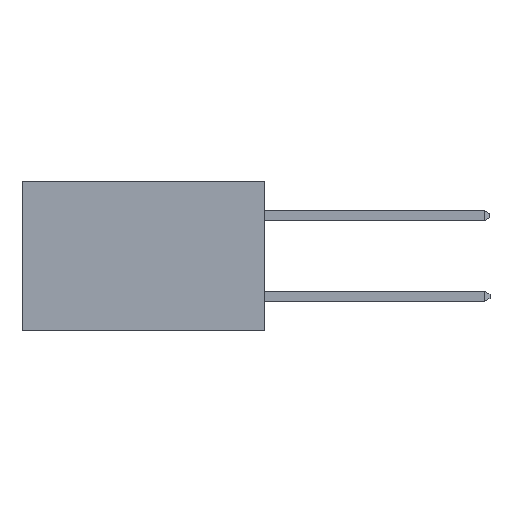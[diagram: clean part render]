
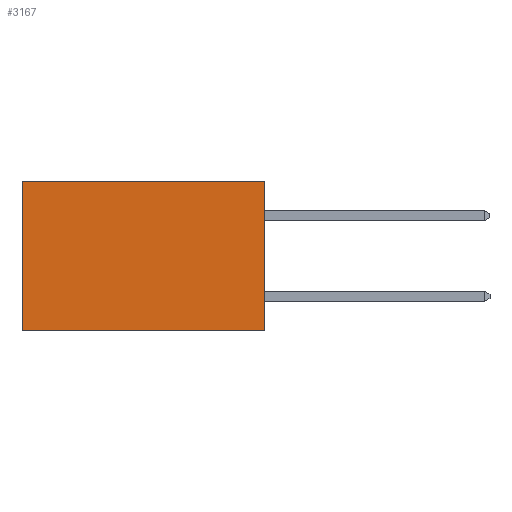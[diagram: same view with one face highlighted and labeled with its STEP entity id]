
A CAD part, left-side view. The second image highlights one B-rep face of the part: STEP entity #3167.
In plain terms, the highlighted planar face has unit normal (-1, 0, 0).
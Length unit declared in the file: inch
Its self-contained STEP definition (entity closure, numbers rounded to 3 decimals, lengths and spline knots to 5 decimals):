
#924 = CARTESIAN_POINT ( 'NONE',  ( 0.2615, 0., -0.37 ) ) ;
#979 = VERTEX_POINT ( 'NONE', #7619 ) ;
#1154 = CARTESIAN_POINT ( 'NONE',  ( 0.2615, 0., -0.37 ) ) ;
#1289 = ORIENTED_EDGE ( 'NONE', *, *, #2136, .F. ) ;
#1330 = DIRECTION ( 'NONE',  ( 0., 1., 0. ) ) ;
#1347 = VECTOR ( 'NONE', #8367, 39.37008 ) ;
#1415 = EDGE_CURVE ( 'NONE', #9553, #979, #8487, .T. ) ;
#1948 = VECTOR ( 'NONE', #10229, 39.37008 ) ;
#2136 = EDGE_CURVE ( 'NONE', #9553, #9776, #6276, .T. ) ;
#2620 = DIRECTION ( 'NONE',  ( 0., 0., -1. ) ) ;
#2632 = DIRECTION ( 'NONE',  ( 1., 0., 0. ) ) ;
#2644 = CARTESIAN_POINT ( 'NONE',  ( 0.2615, 0., -0.37 ) ) ;
#2658 = AXIS2_PLACEMENT_3D ( 'NONE', #2644, #2632, #2620 ) ;
#2882 = VECTOR ( 'NONE', #8326, 39.37008 ) ;
#3016 = ORIENTED_EDGE ( 'NONE', *, *, #4166, .T. ) ;
#3062 = PLANE ( 'NONE',  #2658 ) ;
#3167 = ADVANCED_FACE ( 'NONE', ( #7702 ), #3062, .F. ) ;
#3366 = EDGE_LOOP ( 'NONE', ( #3016, #5436, #1289, #9720 ) ) ;
#3590 = LINE ( 'NONE', #1154, #7774 ) ;
#3872 = LINE ( 'NONE', #8493, #1347 ) ;
#4166 = EDGE_CURVE ( 'NONE', #979, #9088, #3872, .T. ) ;
#5299 = CARTESIAN_POINT ( 'NONE',  ( 0.2615, 0., 0. ) ) ;
#5436 = ORIENTED_EDGE ( 'NONE', *, *, #6499, .F. ) ;
#6276 = LINE ( 'NONE', #924, #1948 ) ;
#6499 = EDGE_CURVE ( 'NONE', #9776, #9088, #3590, .T. ) ;
#7619 = CARTESIAN_POINT ( 'NONE',  ( 0.2615, 0.6, 0. ) ) ;
#7702 = FACE_OUTER_BOUND ( 'NONE', #3366, .T. ) ;
#7774 = VECTOR ( 'NONE', #1330, 39.37008 ) ;
#7931 = CARTESIAN_POINT ( 'NONE',  ( 0.2615, 0.6, -0.37 ) ) ;
#8326 = DIRECTION ( 'NONE',  ( 0., 1., 0. ) ) ;
#8367 = DIRECTION ( 'NONE',  ( 0., 0., -1. ) ) ;
#8399 = CARTESIAN_POINT ( 'NONE',  ( 0.2615, 0., 0. ) ) ;
#8487 = LINE ( 'NONE', #8399, #2882 ) ;
#8493 = CARTESIAN_POINT ( 'NONE',  ( 0.2615, 0.6, -0.37 ) ) ;
#9088 = VERTEX_POINT ( 'NONE', #7931 ) ;
#9553 = VERTEX_POINT ( 'NONE', #5299 ) ;
#9720 = ORIENTED_EDGE ( 'NONE', *, *, #1415, .T. ) ;
#9776 = VERTEX_POINT ( 'NONE', #10006 ) ;
#10006 = CARTESIAN_POINT ( 'NONE',  ( 0.2615, 0., -0.37 ) ) ;
#10229 = DIRECTION ( 'NONE',  ( 0., 0., -1. ) ) ;
